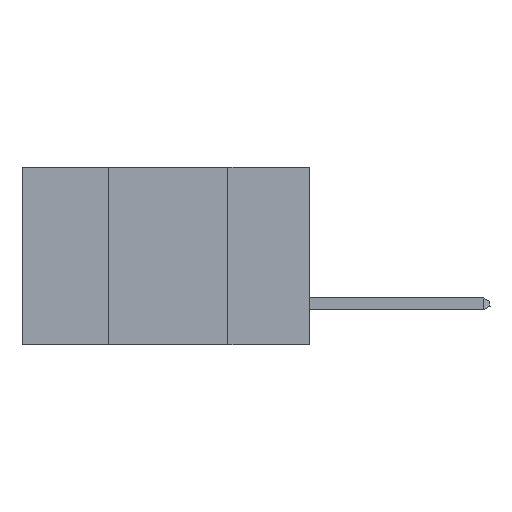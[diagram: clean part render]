
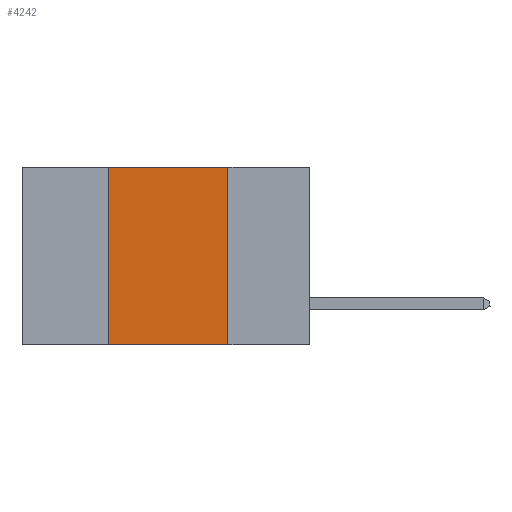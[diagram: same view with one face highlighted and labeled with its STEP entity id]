
A CAD part, left-side view. The second image highlights one B-rep face of the part: STEP entity #4242.
In plain terms, the highlighted planar face has unit normal (-1, 0, 0).
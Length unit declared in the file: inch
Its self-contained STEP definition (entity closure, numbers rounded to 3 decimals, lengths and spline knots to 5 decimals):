
#98 = LINE ( 'NONE', #3193, #7472 ) ;
#729 = ORIENTED_EDGE ( 'NONE', *, *, #9769, .F. ) ;
#1765 = DIRECTION ( 'NONE',  ( 0., -1., 0. ) ) ;
#1968 = VERTEX_POINT ( 'NONE', #11418 ) ;
#3126 = DIRECTION ( 'NONE',  ( 1., 0., 0. ) ) ;
#3193 = CARTESIAN_POINT ( 'NONE',  ( 0., 0.6, 0. ) ) ;
#3483 = EDGE_CURVE ( 'NONE', #1968, #8644, #3654, .T. ) ;
#3654 = LINE ( 'NONE', #13862, #9589 ) ;
#4242 = ADVANCED_FACE ( 'NONE', ( #14254 ), #7526, .F. ) ;
#4386 = EDGE_CURVE ( 'NONE', #4559, #7404, #98, .T. ) ;
#4407 = CARTESIAN_POINT ( 'NONE',  ( 0., 0.42, 0. ) ) ;
#4559 = VERTEX_POINT ( 'NONE', #4407 ) ;
#5322 = CARTESIAN_POINT ( 'NONE',  ( 0., 0.6, 0. ) ) ;
#6165 = LINE ( 'NONE', #14231, #6327 ) ;
#6327 = VECTOR ( 'NONE', #8029, 39.37008 ) ;
#7404 = VERTEX_POINT ( 'NONE', #12465 ) ;
#7472 = VECTOR ( 'NONE', #1765, 39.37008 ) ;
#7526 = PLANE ( 'NONE',  #10254 ) ;
#7845 = DIRECTION ( 'NONE',  ( 0., 0., -1. ) ) ;
#8029 = DIRECTION ( 'NONE',  ( 0., 0., -1. ) ) ;
#8104 = CARTESIAN_POINT ( 'NONE',  ( 0., 0.17, -0.37 ) ) ;
#8644 = VERTEX_POINT ( 'NONE', #8104 ) ;
#9569 = DIRECTION ( 'NONE',  ( 0., -1., 0. ) ) ;
#9589 = VECTOR ( 'NONE', #9569, 39.37008 ) ;
#9769 = EDGE_CURVE ( 'NONE', #7404, #8644, #6165, .T. ) ;
#9803 = ORIENTED_EDGE ( 'NONE', *, *, #3483, .T. ) ;
#10254 = AXIS2_PLACEMENT_3D ( 'NONE', #5322, #3126, #7845 ) ;
#10265 = ORIENTED_EDGE ( 'NONE', *, *, #12274, .F. ) ;
#10269 = ORIENTED_EDGE ( 'NONE', *, *, #4386, .F. ) ;
#10694 = EDGE_LOOP ( 'NONE', ( #729, #10269, #10265, #9803 ) ) ;
#10741 = VECTOR ( 'NONE', #11226, 39.37008 ) ;
#11226 = DIRECTION ( 'NONE',  ( 0., 0., 1. ) ) ;
#11418 = CARTESIAN_POINT ( 'NONE',  ( 0., 0.42, -0.37 ) ) ;
#11428 = CARTESIAN_POINT ( 'NONE',  ( 0., 0.42, 0. ) ) ;
#12274 = EDGE_CURVE ( 'NONE', #1968, #4559, #14403, .T. ) ;
#12465 = CARTESIAN_POINT ( 'NONE',  ( 0., 0.17, 0. ) ) ;
#13862 = CARTESIAN_POINT ( 'NONE',  ( 0., 0.6, -0.37 ) ) ;
#14231 = CARTESIAN_POINT ( 'NONE',  ( 0., 0.17, 0. ) ) ;
#14254 = FACE_OUTER_BOUND ( 'NONE', #10694, .T. ) ;
#14403 = LINE ( 'NONE', #11428, #10741 ) ;
